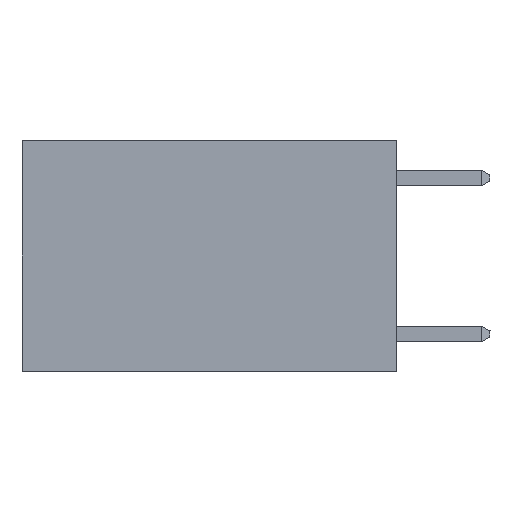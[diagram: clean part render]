
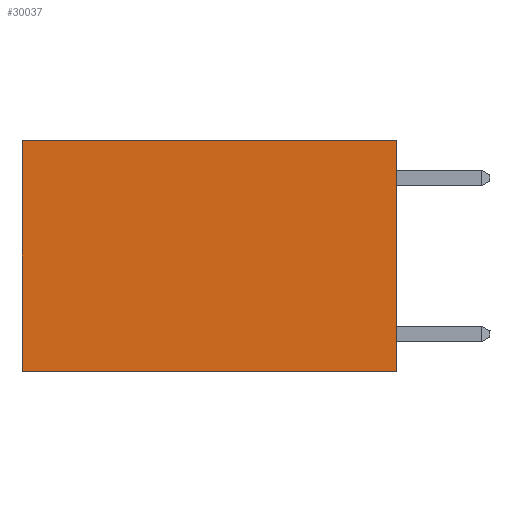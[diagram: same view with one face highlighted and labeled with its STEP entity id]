
A CAD part, left-side view. The second image highlights one B-rep face of the part: STEP entity #30037.
In plain terms, the highlighted planar face has unit normal (-1, 0, 0).
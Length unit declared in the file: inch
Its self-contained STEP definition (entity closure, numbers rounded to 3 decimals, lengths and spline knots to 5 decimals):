
#1322 = DIRECTION ( 'NONE',  ( 0., 1., 0. ) ) ;
#2210 = VECTOR ( 'NONE', #29303, 39.37008 ) ;
#3096 = CARTESIAN_POINT ( 'NONE',  ( 0.2625, 0., 0. ) ) ;
#4670 = EDGE_CURVE ( 'NONE', #25486, #20759, #6000, .T. ) ;
#4863 = CARTESIAN_POINT ( 'NONE',  ( 0.2625, 0., 0. ) ) ;
#5811 = VECTOR ( 'NONE', #6102, 39.37008 ) ;
#6000 = LINE ( 'NONE', #30174, #5811 ) ;
#6102 = DIRECTION ( 'NONE',  ( 0., 0., -1. ) ) ;
#8006 = LINE ( 'NONE', #12263, #2210 ) ;
#8636 = CARTESIAN_POINT ( 'NONE',  ( 0.2625, 0., 0. ) ) ;
#9084 = EDGE_CURVE ( 'NONE', #9712, #23773, #18047, .T. ) ;
#9688 = CARTESIAN_POINT ( 'NONE',  ( 0.2625, 0.6, -0.37 ) ) ;
#9712 = VERTEX_POINT ( 'NONE', #3096 ) ;
#9724 = CARTESIAN_POINT ( 'NONE',  ( 0.2625, 0.6, 0. ) ) ;
#10061 = PLANE ( 'NONE',  #13180 ) ;
#11694 = EDGE_LOOP ( 'NONE', ( #28265, #13258, #27765, #17730 ) ) ;
#12263 = CARTESIAN_POINT ( 'NONE',  ( 0.2625, 0., -0.37 ) ) ;
#13180 = AXIS2_PLACEMENT_3D ( 'NONE', #27069, #29425, #15003 ) ;
#13258 = ORIENTED_EDGE ( 'NONE', *, *, #21775, .F. ) ;
#14304 = FACE_OUTER_BOUND ( 'NONE', #11694, .T. ) ;
#15003 = DIRECTION ( 'NONE',  ( 0., 0., -1. ) ) ;
#17436 = CARTESIAN_POINT ( 'NONE',  ( 0.2625, 0., -0.37 ) ) ;
#17445 = EDGE_CURVE ( 'NONE', #9712, #25486, #31087, .T. ) ;
#17730 = ORIENTED_EDGE ( 'NONE', *, *, #17445, .T. ) ;
#18047 = LINE ( 'NONE', #4863, #29304 ) ;
#20759 = VERTEX_POINT ( 'NONE', #9688 ) ;
#21775 = EDGE_CURVE ( 'NONE', #23773, #20759, #8006, .T. ) ;
#23773 = VERTEX_POINT ( 'NONE', #17436 ) ;
#24336 = DIRECTION ( 'NONE',  ( 0., 0., -1. ) ) ;
#24878 = VECTOR ( 'NONE', #1322, 39.37008 ) ;
#25486 = VERTEX_POINT ( 'NONE', #9724 ) ;
#27069 = CARTESIAN_POINT ( 'NONE',  ( 0.2625, 0., 0. ) ) ;
#27765 = ORIENTED_EDGE ( 'NONE', *, *, #9084, .F. ) ;
#28265 = ORIENTED_EDGE ( 'NONE', *, *, #4670, .T. ) ;
#29303 = DIRECTION ( 'NONE',  ( 0., 1., 0. ) ) ;
#29304 = VECTOR ( 'NONE', #24336, 39.37008 ) ;
#29425 = DIRECTION ( 'NONE',  ( 1., 0., 0. ) ) ;
#30037 = ADVANCED_FACE ( 'NONE', ( #14304 ), #10061, .F. ) ;
#30174 = CARTESIAN_POINT ( 'NONE',  ( 0.2625, 0.6, 0. ) ) ;
#31087 = LINE ( 'NONE', #8636, #24878 ) ;
